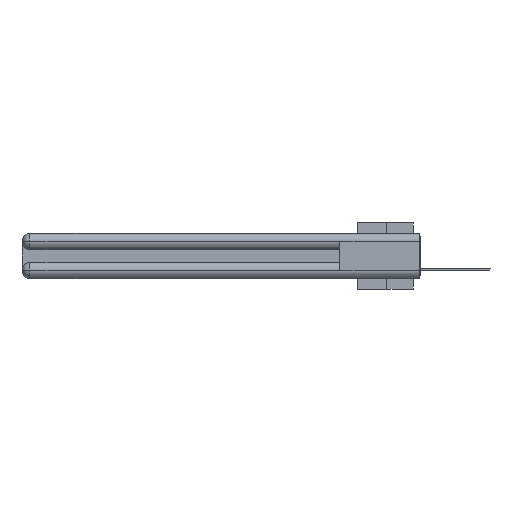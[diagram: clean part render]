
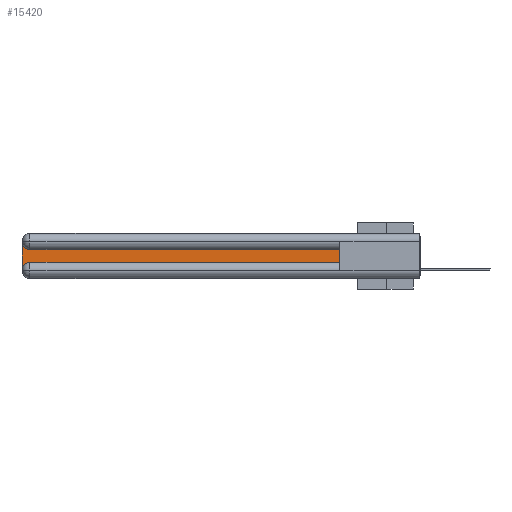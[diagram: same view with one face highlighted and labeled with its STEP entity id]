
A CAD part, left-side view. The second image highlights one B-rep face of the part: STEP entity #15420.
In plain terms, the highlighted planar face has unit normal (-1, 0, 0).
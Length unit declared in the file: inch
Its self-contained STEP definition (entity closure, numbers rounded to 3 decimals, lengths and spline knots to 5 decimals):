
#63 = LINE ( 'NONE', #14447, #29172 ) ;
#610 = CARTESIAN_POINT ( 'NONE',  ( 0.075, 2.94, -0.2175 ) ) ;
#732 = CARTESIAN_POINT ( 'NONE',  ( 0.075, 2.94, -0.0625 ) ) ;
#1059 = DIRECTION ( 'NONE',  ( 0., 0., -1. ) ) ;
#1397 = LINE ( 'NONE', #19361, #6515 ) ;
#1670 = LINE ( 'NONE', #22040, #19821 ) ;
#2197 = ORIENTED_EDGE ( 'NONE', *, *, #24562, .T. ) ;
#2308 = CIRCLE ( 'NONE', #17078, 0.06 ) ;
#3278 = CARTESIAN_POINT ( 'NONE',  ( 0.075, 3., -0.2175 ) ) ;
#4737 = VERTEX_POINT ( 'NONE', #10814 ) ;
#5847 = VERTEX_POINT ( 'NONE', #34671 ) ;
#6011 = ORIENTED_EDGE ( 'NONE', *, *, #20902, .T. ) ;
#6278 = ORIENTED_EDGE ( 'NONE', *, *, #28469, .T. ) ;
#6515 = VECTOR ( 'NONE', #30253, 39.37008 ) ;
#9174 = DIRECTION ( 'NONE',  ( 0., 0., -1. ) ) ;
#9370 = PLANE ( 'NONE',  #28630 ) ;
#10712 = ORIENTED_EDGE ( 'NONE', *, *, #25976, .T. ) ;
#10814 = CARTESIAN_POINT ( 'NONE',  ( 0.075, 3., -0.0625 ) ) ;
#11515 = CIRCLE ( 'NONE', #26829, 0.06 ) ;
#14098 = DIRECTION ( 'NONE',  ( 0., 0., -1. ) ) ;
#14331 = DIRECTION ( 'NONE',  ( 0., -1., 0. ) ) ;
#14445 = VERTEX_POINT ( 'NONE', #23050 ) ;
#14447 = CARTESIAN_POINT ( 'NONE',  ( 0.075, 0.6, -0.2175 ) ) ;
#15420 = ADVANCED_FACE ( 'NONE', ( #33734 ), #9370, .F. ) ;
#16399 = EDGE_LOOP ( 'NONE', ( #6011, #32048, #6278, #33089, #10712, #2197 ) ) ;
#16942 = DIRECTION ( 'NONE',  ( 1., 0., 0. ) ) ;
#17078 = AXIS2_PLACEMENT_3D ( 'NONE', #732, #16942, #9174 ) ;
#17382 = DIRECTION ( 'NONE',  ( 1., 0., 0. ) ) ;
#17632 = CARTESIAN_POINT ( 'NONE',  ( 0.075, 3., -0.1225 ) ) ;
#19361 = CARTESIAN_POINT ( 'NONE',  ( 0.075, 0.6, -0.2175 ) ) ;
#19821 = VECTOR ( 'NONE', #22269, 39.37008 ) ;
#20902 = EDGE_CURVE ( 'NONE', #5847, #29576, #1670, .T. ) ;
#21418 = VERTEX_POINT ( 'NONE', #610 ) ;
#21457 = CARTESIAN_POINT ( 'NONE',  ( 0.075, 2.94, -0.1225 ) ) ;
#22040 = CARTESIAN_POINT ( 'NONE',  ( 0.075, 0.6, -0.1225 ) ) ;
#22269 = DIRECTION ( 'NONE',  ( 0., 1., 0. ) ) ;
#22374 = VECTOR ( 'NONE', #14098, 39.37008 ) ;
#23050 = CARTESIAN_POINT ( 'NONE',  ( 0.075, 0.6, -0.2175 ) ) ;
#23205 = DIRECTION ( 'NONE',  ( 0., 0., -1. ) ) ;
#24562 = EDGE_CURVE ( 'NONE', #14445, #5847, #1397, .T. ) ;
#24615 = VERTEX_POINT ( 'NONE', #27462 ) ;
#25976 = EDGE_CURVE ( 'NONE', #21418, #14445, #63, .T. ) ;
#26829 = AXIS2_PLACEMENT_3D ( 'NONE', #34238, #28921, #23205 ) ;
#27297 = EDGE_CURVE ( 'NONE', #24615, #21418, #11515, .T. ) ;
#27462 = CARTESIAN_POINT ( 'NONE',  ( 0.075, 3., -0.2775 ) ) ;
#28469 = EDGE_CURVE ( 'NONE', #4737, #24615, #28690, .T. ) ;
#28630 = AXIS2_PLACEMENT_3D ( 'NONE', #17632, #17382, #1059 ) ;
#28690 = LINE ( 'NONE', #3278, #22374 ) ;
#28921 = DIRECTION ( 'NONE',  ( 1., 0., 0. ) ) ;
#29172 = VECTOR ( 'NONE', #14331, 39.37008 ) ;
#29576 = VERTEX_POINT ( 'NONE', #21457 ) ;
#30253 = DIRECTION ( 'NONE',  ( 0., 0., 1. ) ) ;
#32048 = ORIENTED_EDGE ( 'NONE', *, *, #34373, .T. ) ;
#33089 = ORIENTED_EDGE ( 'NONE', *, *, #27297, .T. ) ;
#33734 = FACE_OUTER_BOUND ( 'NONE', #16399, .T. ) ;
#34238 = CARTESIAN_POINT ( 'NONE',  ( 0.075, 2.94, -0.2775 ) ) ;
#34373 = EDGE_CURVE ( 'NONE', #29576, #4737, #2308, .T. ) ;
#34671 = CARTESIAN_POINT ( 'NONE',  ( 0.075, 0.6, -0.1225 ) ) ;
